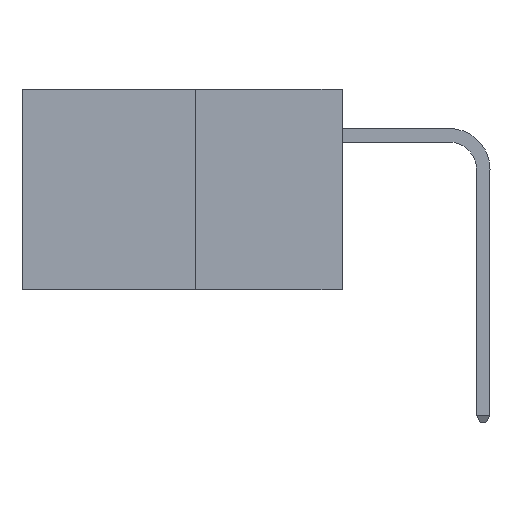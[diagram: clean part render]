
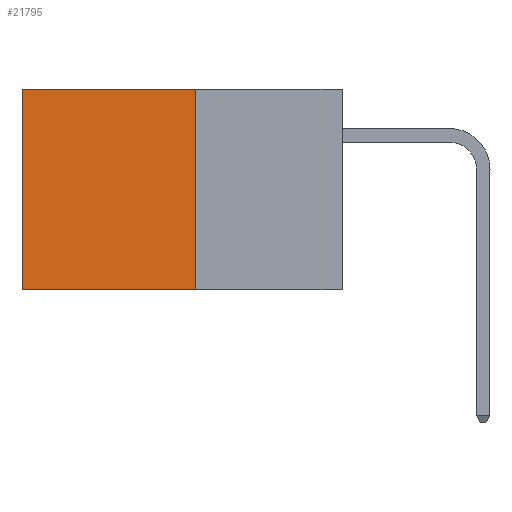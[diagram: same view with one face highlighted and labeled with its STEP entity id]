
A CAD part, left-side view. The second image highlights one B-rep face of the part: STEP entity #21795.
In plain terms, the highlighted planar face has unit normal (-1, 0, 0).
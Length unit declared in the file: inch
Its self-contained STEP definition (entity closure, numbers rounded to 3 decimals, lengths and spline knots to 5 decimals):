
#15 = ORIENTED_EDGE ( 'NONE', *, *, #6489, .T. ) ;
#340 = VECTOR ( 'NONE', #18262, 39.37008 ) ;
#356 = VERTEX_POINT ( 'NONE', #2436 ) ;
#577 = CARTESIAN_POINT ( 'NONE',  ( 0.277, 0.27, -0.37 ) ) ;
#1333 = ORIENTED_EDGE ( 'NONE', *, *, #21765, .F. ) ;
#1858 = DIRECTION ( 'NONE',  ( 0., 0., -1. ) ) ;
#2436 = CARTESIAN_POINT ( 'NONE',  ( 0.277, 0.59, -0.37 ) ) ;
#3021 = FACE_OUTER_BOUND ( 'NONE', #10096, .T. ) ;
#3612 = DIRECTION ( 'NONE',  ( 0., 0., -1. ) ) ;
#3713 = DIRECTION ( 'NONE',  ( 0., 0., -1. ) ) ;
#4014 = CARTESIAN_POINT ( 'NONE',  ( 0.277, 0.59, -0.37 ) ) ;
#4831 = LINE ( 'NONE', #4014, #23691 ) ;
#5354 = CARTESIAN_POINT ( 'NONE',  ( 0.277, 0.27, 0. ) ) ;
#5407 = CARTESIAN_POINT ( 'NONE',  ( 0.277, 0.27, -0.37 ) ) ;
#6489 = EDGE_CURVE ( 'NONE', #13856, #356, #4831, .T. ) ;
#7918 = VECTOR ( 'NONE', #3612, 39.37008 ) ;
#7957 = AXIS2_PLACEMENT_3D ( 'NONE', #11015, #12907, #1858 ) ;
#8514 = LINE ( 'NONE', #13224, #7918 ) ;
#8562 = CARTESIAN_POINT ( 'NONE',  ( 0.277, 0.27, 0. ) ) ;
#9165 = PLANE ( 'NONE',  #7957 ) ;
#10096 = EDGE_LOOP ( 'NONE', ( #15, #12657, #1333, #14855 ) ) ;
#11015 = CARTESIAN_POINT ( 'NONE',  ( 0.277, 0.27, -0.37 ) ) ;
#12164 = VERTEX_POINT ( 'NONE', #577 ) ;
#12264 = VERTEX_POINT ( 'NONE', #8562 ) ;
#12657 = ORIENTED_EDGE ( 'NONE', *, *, #15440, .F. ) ;
#12907 = DIRECTION ( 'NONE',  ( 1., 0., 0. ) ) ;
#13224 = CARTESIAN_POINT ( 'NONE',  ( 0.277, 0.27, -0.37 ) ) ;
#13856 = VERTEX_POINT ( 'NONE', #21065 ) ;
#14717 = DIRECTION ( 'NONE',  ( 0., 1., 0. ) ) ;
#14855 = ORIENTED_EDGE ( 'NONE', *, *, #18086, .T. ) ;
#15440 = EDGE_CURVE ( 'NONE', #12164, #356, #20383, .T. ) ;
#15523 = VECTOR ( 'NONE', #14717, 39.37008 ) ;
#18086 = EDGE_CURVE ( 'NONE', #12264, #13856, #19334, .T. ) ;
#18262 = DIRECTION ( 'NONE',  ( 0., 1., 0. ) ) ;
#19334 = LINE ( 'NONE', #5354, #340 ) ;
#20383 = LINE ( 'NONE', #5407, #15523 ) ;
#21065 = CARTESIAN_POINT ( 'NONE',  ( 0.277, 0.59, 0. ) ) ;
#21765 = EDGE_CURVE ( 'NONE', #12264, #12164, #8514, .T. ) ;
#21795 = ADVANCED_FACE ( 'NONE', ( #3021 ), #9165, .F. ) ;
#23691 = VECTOR ( 'NONE', #3713, 39.37008 ) ;
